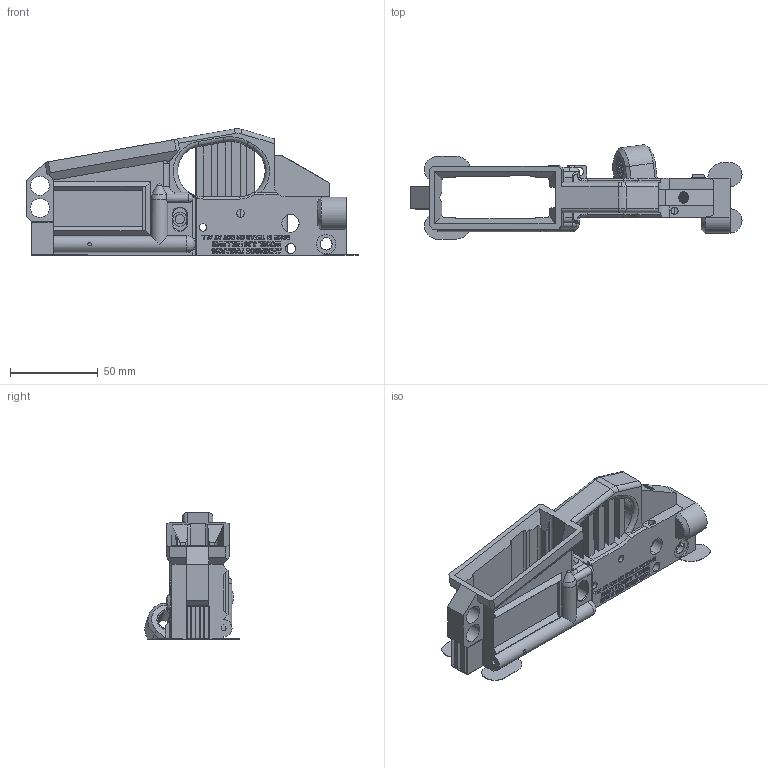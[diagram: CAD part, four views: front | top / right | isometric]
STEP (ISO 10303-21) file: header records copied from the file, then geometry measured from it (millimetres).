
FILE_DESCRIPTION (( 'STEP AP203' ), '1' );
FILE_NAME ('AF-HF-LR-PRT-001-STEP_FULL_FUCKING_AUTO_EDITION.STEP', '2020-10-04T16:47:35', ( '' ), ( '' ), 'SwSTEP 2.0', 'SolidWorks 2018', '' );
FILE_SCHEMA (( 'CONFIG_CONTROL_DESIGN' ));
Products named in the file (1): AF-HF-LR-PRT-001-STEP_FULL_FUCKING_AUTO_EDITION
Bounding box: 189.59 x 53.91 x 72.31 mm (x, y, z)
Volume: 100233.4 mm3; surface area: 78309.1 mm2
Topology: 1 solids, 1 shells, 2758 faces, 7698 edges, 5080 vertices
Faces by surface type: plane 1911, bspline 544, cylinder 260, torus 22, cone 17, sphere 4
Entity records: 165889 total; most frequent: CARTESIAN_POINT 99757, ORIENTED_EDGE 15384, DIRECTION 11063, EDGE_CURVE 7692, VECTOR 5649, LINE 5649, VERTEX_POINT 5079, EDGE_LOOP 2973
